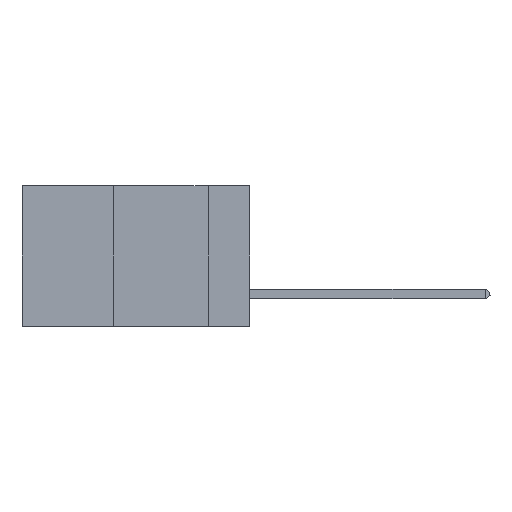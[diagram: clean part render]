
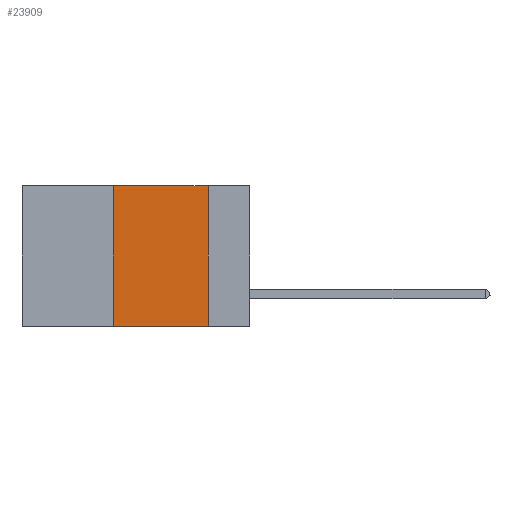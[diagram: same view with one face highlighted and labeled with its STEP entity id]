
A CAD part, left-side view. The second image highlights one B-rep face of the part: STEP entity #23909.
In plain terms, the highlighted planar face has unit normal (-1, 0, 0).
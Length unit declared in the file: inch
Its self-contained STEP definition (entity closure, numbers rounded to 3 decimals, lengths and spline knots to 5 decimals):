
#200 = LINE ( 'NONE', #22684, #4322 ) ;
#460 = VECTOR ( 'NONE', #10630, 39.37008 ) ;
#2043 = VECTOR ( 'NONE', #10855, 39.37008 ) ;
#4322 = VECTOR ( 'NONE', #5726, 39.37008 ) ;
#4651 = EDGE_CURVE ( 'NONE', #16290, #6108, #6561, .T. ) ;
#5431 = EDGE_CURVE ( 'NONE', #7989, #12667, #18168, .T. ) ;
#5723 = ORIENTED_EDGE ( 'NONE', *, *, #5431, .F. ) ;
#5726 = DIRECTION ( 'NONE',  ( 0., -1., 0. ) ) ;
#6108 = VERTEX_POINT ( 'NONE', #8117 ) ;
#6561 = LINE ( 'NONE', #23982, #27622 ) ;
#7159 = EDGE_LOOP ( 'NONE', ( #28791, #7526, #5723, #23227 ) ) ;
#7526 = ORIENTED_EDGE ( 'NONE', *, *, #14518, .F. ) ;
#7989 = VERTEX_POINT ( 'NONE', #22902 ) ;
#8117 = CARTESIAN_POINT ( 'NONE',  ( 0., 0.11, -0.37 ) ) ;
#8181 = CARTESIAN_POINT ( 'NONE',  ( 0., 0.6, -0.37 ) ) ;
#9540 = DIRECTION ( 'NONE',  ( 1., 0., 0. ) ) ;
#10195 = DIRECTION ( 'NONE',  ( 0., 0., -1. ) ) ;
#10630 = DIRECTION ( 'NONE',  ( 0., -1., 0. ) ) ;
#10855 = DIRECTION ( 'NONE',  ( 0., 0., 1. ) ) ;
#11985 = FACE_OUTER_BOUND ( 'NONE', #7159, .T. ) ;
#12667 = VERTEX_POINT ( 'NONE', #16357 ) ;
#12980 = EDGE_CURVE ( 'NONE', #7989, #6108, #23000, .T. ) ;
#14518 = EDGE_CURVE ( 'NONE', #12667, #16290, #200, .T. ) ;
#16062 = CARTESIAN_POINT ( 'NONE',  ( 0., 0.36, 0. ) ) ;
#16290 = VERTEX_POINT ( 'NONE', #27519 ) ;
#16357 = CARTESIAN_POINT ( 'NONE',  ( 0., 0.36, 0. ) ) ;
#18168 = LINE ( 'NONE', #16062, #2043 ) ;
#19482 = PLANE ( 'NONE',  #22471 ) ;
#22471 = AXIS2_PLACEMENT_3D ( 'NONE', #31843, #9540, #10195 ) ;
#22684 = CARTESIAN_POINT ( 'NONE',  ( 0., 0.6, 0. ) ) ;
#22902 = CARTESIAN_POINT ( 'NONE',  ( 0., 0.36, -0.37 ) ) ;
#23000 = LINE ( 'NONE', #8181, #460 ) ;
#23227 = ORIENTED_EDGE ( 'NONE', *, *, #12980, .T. ) ;
#23909 = ADVANCED_FACE ( 'NONE', ( #11985 ), #19482, .F. ) ;
#23982 = CARTESIAN_POINT ( 'NONE',  ( 0., 0.11, 0. ) ) ;
#26439 = DIRECTION ( 'NONE',  ( 0., 0., -1. ) ) ;
#27519 = CARTESIAN_POINT ( 'NONE',  ( 0., 0.11, 0. ) ) ;
#27622 = VECTOR ( 'NONE', #26439, 39.37008 ) ;
#28791 = ORIENTED_EDGE ( 'NONE', *, *, #4651, .F. ) ;
#31843 = CARTESIAN_POINT ( 'NONE',  ( 0., 0.6, 0. ) ) ;
